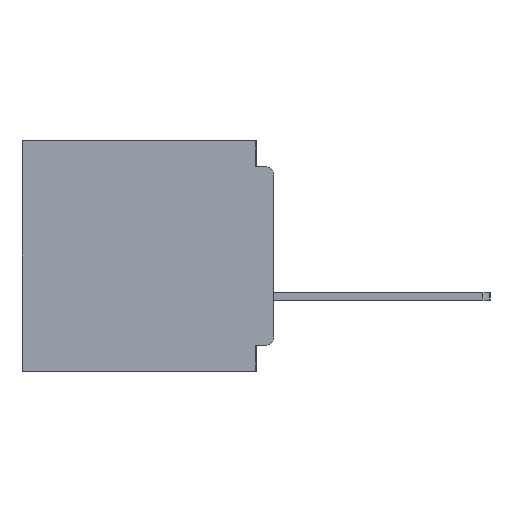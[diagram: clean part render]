
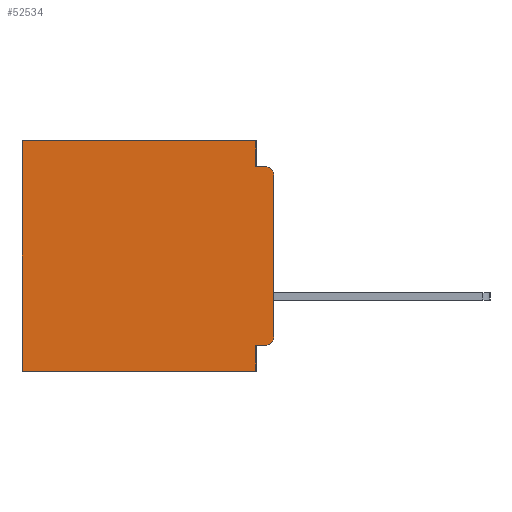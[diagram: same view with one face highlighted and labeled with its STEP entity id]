
A CAD part, left-side view. The second image highlights one B-rep face of the part: STEP entity #52534.
In plain terms, the highlighted planar face has unit normal (-1, 0, 0).
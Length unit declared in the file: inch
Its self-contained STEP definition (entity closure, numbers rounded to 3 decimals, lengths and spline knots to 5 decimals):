
#280 = CARTESIAN_POINT ( 'NONE',  ( 0.3, 0., -0.34 ) ) ;
#841 = LINE ( 'NONE', #29830, #10523 ) ;
#1705 = VERTEX_POINT ( 'NONE', #10992 ) ;
#1996 = CARTESIAN_POINT ( 'NONE',  ( 0.3, 0.437, -0.4 ) ) ;
#2960 = ORIENTED_EDGE ( 'NONE', *, *, #15706, .T. ) ;
#3088 = VECTOR ( 'NONE', #9761, 39.37008 ) ;
#3660 = EDGE_CURVE ( 'NONE', #1705, #48258, #841, .T. ) ;
#3809 = CARTESIAN_POINT ( 'NONE',  ( 0.3, 0.015, -0.34 ) ) ;
#4378 = LINE ( 'NONE', #5632, #3088 ) ;
#4560 = CARTESIAN_POINT ( 'NONE',  ( 0.3, 0.015, -0.06 ) ) ;
#5632 = CARTESIAN_POINT ( 'NONE',  ( 0.3, 0., -0.4 ) ) ;
#6028 = DIRECTION ( 'NONE',  ( 0., 1., 0. ) ) ;
#6634 = DIRECTION ( 'NONE',  ( 0., 1., 0. ) ) ;
#7737 = ORIENTED_EDGE ( 'NONE', *, *, #13277, .F. ) ;
#7979 = DIRECTION ( 'NONE',  ( 0., 0., -1. ) ) ;
#7987 = LINE ( 'NONE', #31291, #27290 ) ;
#8729 = DIRECTION ( 'NONE',  ( 0., 0., -1. ) ) ;
#8915 = LINE ( 'NONE', #45450, #51373 ) ;
#9706 = VERTEX_POINT ( 'NONE', #21843 ) ;
#9761 = DIRECTION ( 'NONE',  ( 0., 0., -1. ) ) ;
#9891 = AXIS2_PLACEMENT_3D ( 'NONE', #3809, #32630, #7979 ) ;
#9936 = EDGE_LOOP ( 'NONE', ( #7737, #49643, #39110, #15357, #2960, #11154, #32788, #47353, #51117, #31561 ) ) ;
#10523 = VECTOR ( 'NONE', #42238, 39.37008 ) ;
#10992 = CARTESIAN_POINT ( 'NONE',  ( 0.3, 0.015, -0.355 ) ) ;
#11154 = ORIENTED_EDGE ( 'NONE', *, *, #24684, .T. ) ;
#13277 = EDGE_CURVE ( 'NONE', #35787, #49092, #4378, .T. ) ;
#15278 = CIRCLE ( 'NONE', #23417, 0.015 ) ;
#15357 = ORIENTED_EDGE ( 'NONE', *, *, #24156, .F. ) ;
#15706 = EDGE_CURVE ( 'NONE', #25132, #9706, #25472, .T. ) ;
#15981 = EDGE_CURVE ( 'NONE', #1705, #49092, #23502, .T. ) ;
#16657 = DIRECTION ( 'NONE',  ( 0., -1., 0. ) ) ;
#19279 = CARTESIAN_POINT ( 'NONE',  ( 0.3, 0.031, 0. ) ) ;
#19973 = VECTOR ( 'NONE', #20414, 39.37008 ) ;
#20414 = DIRECTION ( 'NONE',  ( 0., 0., -1. ) ) ;
#21843 = CARTESIAN_POINT ( 'NONE',  ( 0.3, 0.437, 0. ) ) ;
#22377 = CARTESIAN_POINT ( 'NONE',  ( 0.3, 0., 0. ) ) ;
#23153 = PLANE ( 'NONE',  #39318 ) ;
#23401 = CARTESIAN_POINT ( 'NONE',  ( 0.3, 0.031, -0.355 ) ) ;
#23417 = AXIS2_PLACEMENT_3D ( 'NONE', #4560, #33360, #8729 ) ;
#23502 = CIRCLE ( 'NONE', #9891, 0.015 ) ;
#24156 = EDGE_CURVE ( 'NONE', #25132, #39298, #49663, .T. ) ;
#24432 = DIRECTION ( 'NONE',  ( 0., 0., -1. ) ) ;
#24684 = EDGE_CURVE ( 'NONE', #9706, #48098, #41875, .T. ) ;
#25132 = VERTEX_POINT ( 'NONE', #19279 ) ;
#25472 = LINE ( 'NONE', #22377, #35146 ) ;
#26487 = VECTOR ( 'NONE', #24432, 39.37008 ) ;
#27140 = CARTESIAN_POINT ( 'NONE',  ( 0.3, 0., -0.4 ) ) ;
#27290 = VECTOR ( 'NONE', #6634, 39.37008 ) ;
#27318 = DIRECTION ( 'NONE',  ( 0., 0., -1. ) ) ;
#27446 = VECTOR ( 'NONE', #32757, 39.37008 ) ;
#27656 = FACE_OUTER_BOUND ( 'NONE', #9936, .T. ) ;
#29830 = CARTESIAN_POINT ( 'NONE',  ( 0.3, 0., -0.355 ) ) ;
#31291 = CARTESIAN_POINT ( 'NONE',  ( 0.3, 0., -0.4 ) ) ;
#31488 = EDGE_CURVE ( 'NONE', #35787, #43047, #15278, .T. ) ;
#31561 = ORIENTED_EDGE ( 'NONE', *, *, #15981, .T. ) ;
#32576 = CARTESIAN_POINT ( 'NONE',  ( 0.3, 0., -0.06 ) ) ;
#32630 = DIRECTION ( 'NONE',  ( -1., 0., 0. ) ) ;
#32757 = DIRECTION ( 'NONE',  ( 0., 0., -1. ) ) ;
#32788 = ORIENTED_EDGE ( 'NONE', *, *, #48809, .F. ) ;
#33360 = DIRECTION ( 'NONE',  ( -1., 0., 0. ) ) ;
#34408 = CARTESIAN_POINT ( 'NONE',  ( 0.3, 0.015, -0.045 ) ) ;
#35146 = VECTOR ( 'NONE', #6028, 39.37008 ) ;
#35787 = VERTEX_POINT ( 'NONE', #32576 ) ;
#36829 = CARTESIAN_POINT ( 'NONE',  ( 0.3, 0.437, -0.4 ) ) ;
#38374 = LINE ( 'NONE', #44794, #27446 ) ;
#38642 = VERTEX_POINT ( 'NONE', #45258 ) ;
#39110 = ORIENTED_EDGE ( 'NONE', *, *, #46376, .F. ) ;
#39298 = VERTEX_POINT ( 'NONE', #48044 ) ;
#39318 = AXIS2_PLACEMENT_3D ( 'NONE', #27140, #51944, #27318 ) ;
#39444 = EDGE_CURVE ( 'NONE', #48258, #38642, #38374, .T. ) ;
#41875 = LINE ( 'NONE', #36829, #19973 ) ;
#42238 = DIRECTION ( 'NONE',  ( 0., 1., 0. ) ) ;
#43047 = VERTEX_POINT ( 'NONE', #34408 ) ;
#44794 = CARTESIAN_POINT ( 'NONE',  ( 0.3, 0.031, -0.4 ) ) ;
#45258 = CARTESIAN_POINT ( 'NONE',  ( 0.3, 0.031, -0.4 ) ) ;
#45450 = CARTESIAN_POINT ( 'NONE',  ( 0.3, 0., -0.045 ) ) ;
#46376 = EDGE_CURVE ( 'NONE', #39298, #43047, #8915, .T. ) ;
#47353 = ORIENTED_EDGE ( 'NONE', *, *, #39444, .F. ) ;
#48044 = CARTESIAN_POINT ( 'NONE',  ( 0.3, 0.031, -0.045 ) ) ;
#48098 = VERTEX_POINT ( 'NONE', #1996 ) ;
#48258 = VERTEX_POINT ( 'NONE', #23401 ) ;
#48809 = EDGE_CURVE ( 'NONE', #38642, #48098, #7987, .T. ) ;
#49092 = VERTEX_POINT ( 'NONE', #280 ) ;
#49094 = CARTESIAN_POINT ( 'NONE',  ( 0.3, 0.031, 0. ) ) ;
#49643 = ORIENTED_EDGE ( 'NONE', *, *, #31488, .T. ) ;
#49663 = LINE ( 'NONE', #49094, #26487 ) ;
#51117 = ORIENTED_EDGE ( 'NONE', *, *, #3660, .F. ) ;
#51373 = VECTOR ( 'NONE', #16657, 39.37008 ) ;
#51944 = DIRECTION ( 'NONE',  ( 1., 0., 0. ) ) ;
#52534 = ADVANCED_FACE ( 'NONE', ( #27656 ), #23153, .F. ) ;
